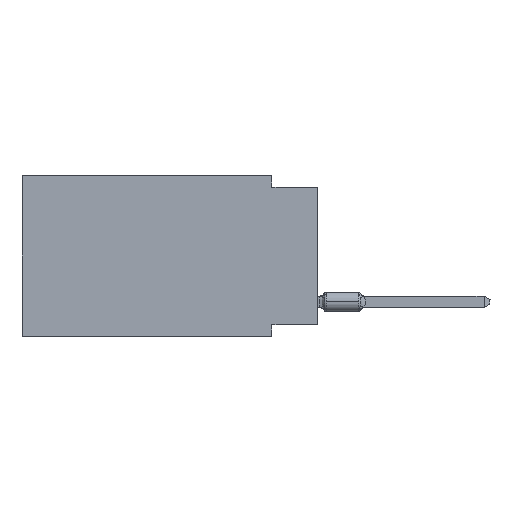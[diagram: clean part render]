
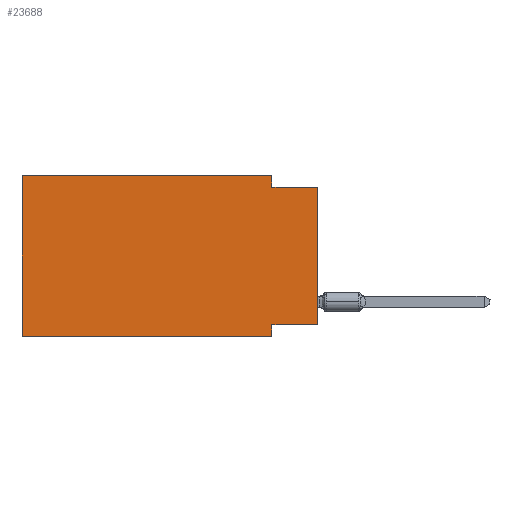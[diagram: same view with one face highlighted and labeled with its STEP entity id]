
A CAD part, left-side view. The second image highlights one B-rep face of the part: STEP entity #23688.
In plain terms, the highlighted planar face has unit normal (-1, 0, 0).
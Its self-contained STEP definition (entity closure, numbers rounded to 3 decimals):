
#523 = LINE ( 'NONE', #6132, #5181 ) ;
#1082 = EDGE_CURVE ( 'NONE', #67866, #2966, #523, .T. ) ;
#2966 = VERTEX_POINT ( 'NONE', #23461 ) ;
#3030 = DIRECTION ( 'NONE',  ( 0., 0., 1. ) ) ;
#3639 = DIRECTION ( 'NONE',  ( 0., 1., 0. ) ) ;
#3882 = VECTOR ( 'NONE', #3030, 1000. ) ;
#4703 = VERTEX_POINT ( 'NONE', #50048 ) ;
#5181 = VECTOR ( 'NONE', #12448, 1000. ) ;
#5575 = EDGE_LOOP ( 'NONE', ( #42075, #51345, #21084, #53376, #48257, #61463, #65077, #19647 ) ) ;
#6132 = CARTESIAN_POINT ( 'NONE',  ( 0., 16.383, 0. ) ) ;
#7193 = AXIS2_PLACEMENT_3D ( 'NONE', #18629, #13002, #58608 ) ;
#8131 = LINE ( 'NONE', #8870, #52992 ) ;
#8870 = CARTESIAN_POINT ( 'NONE',  ( 0., 16.383, 0. ) ) ;
#9353 = CARTESIAN_POINT ( 'NONE',  ( 0., 16.383, 0. ) ) ;
#12448 = DIRECTION ( 'NONE',  ( 0., -1., 0. ) ) ;
#12990 = CARTESIAN_POINT ( 'NONE',  ( 0., 2.54, 0. ) ) ;
#13002 = DIRECTION ( 'NONE',  ( 1., 0., 0. ) ) ;
#13518 = CARTESIAN_POINT ( 'NONE',  ( 0., 2.54, -0.635 ) ) ;
#14638 = EDGE_CURVE ( 'NONE', #60147, #52580, #49582, .T. ) ;
#18629 = CARTESIAN_POINT ( 'NONE',  ( 0., 16.383, 0. ) ) ;
#19647 = ORIENTED_EDGE ( 'NONE', *, *, #14638, .F. ) ;
#21084 = ORIENTED_EDGE ( 'NONE', *, *, #63190, .F. ) ;
#22268 = VECTOR ( 'NONE', #30192, 1000. ) ;
#23461 = CARTESIAN_POINT ( 'NONE',  ( 0., 2.54, 0. ) ) ;
#23688 = ADVANCED_FACE ( 'NONE', ( #30203 ), #41772, .F. ) ;
#24463 = EDGE_CURVE ( 'NONE', #60147, #72265, #46830, .T. ) ;
#25312 = EDGE_CURVE ( 'NONE', #52580, #49282, #31599, .T. ) ;
#26367 = CARTESIAN_POINT ( 'NONE',  ( 0., 2.54, -8.89 ) ) ;
#27574 = CARTESIAN_POINT ( 'NONE',  ( 0., 0., -0.635 ) ) ;
#28910 = VECTOR ( 'NONE', #50147, 1000. ) ;
#30192 = DIRECTION ( 'NONE',  ( 0., 0., -1. ) ) ;
#30203 = FACE_OUTER_BOUND ( 'NONE', #5575, .T. ) ;
#31599 = LINE ( 'NONE', #26367, #43318 ) ;
#32585 = CARTESIAN_POINT ( 'NONE',  ( 0., 16.383, -8.89 ) ) ;
#33531 = DIRECTION ( 'NONE',  ( 0., -1., 0. ) ) ;
#41772 = PLANE ( 'NONE',  #7193 ) ;
#42075 = ORIENTED_EDGE ( 'NONE', *, *, #24463, .T. ) ;
#43318 = VECTOR ( 'NONE', #48796, 1000. ) ;
#46265 = LINE ( 'NONE', #12990, #22268 ) ;
#46830 = LINE ( 'NONE', #58071, #3882 ) ;
#48257 = ORIENTED_EDGE ( 'NONE', *, *, #53502, .F. ) ;
#48796 = DIRECTION ( 'NONE',  ( 0., 0., -1. ) ) ;
#48837 = DIRECTION ( 'NONE',  ( 0., 0., 1. ) ) ;
#49050 = LINE ( 'NONE', #32585, #28910 ) ;
#49282 = VERTEX_POINT ( 'NONE', #66206 ) ;
#49582 = LINE ( 'NONE', #72388, #60807 ) ;
#50048 = CARTESIAN_POINT ( 'NONE',  ( 0., 16.383, -8.89 ) ) ;
#50147 = DIRECTION ( 'NONE',  ( 0., -1., 0. ) ) ;
#51345 = ORIENTED_EDGE ( 'NONE', *, *, #71925, .F. ) ;
#52580 = VERTEX_POINT ( 'NONE', #55951 ) ;
#52992 = VECTOR ( 'NONE', #48837, 1000. ) ;
#53376 = ORIENTED_EDGE ( 'NONE', *, *, #1082, .F. ) ;
#53502 = EDGE_CURVE ( 'NONE', #4703, #67866, #8131, .T. ) ;
#55951 = CARTESIAN_POINT ( 'NONE',  ( 0., 2.54, -8.255 ) ) ;
#56368 = VECTOR ( 'NONE', #33531, 1000. ) ;
#57340 = VERTEX_POINT ( 'NONE', #13518 ) ;
#58071 = CARTESIAN_POINT ( 'NONE',  ( 0., 0., 0. ) ) ;
#58092 = EDGE_CURVE ( 'NONE', #4703, #49282, #49050, .T. ) ;
#58608 = DIRECTION ( 'NONE',  ( 0., 0., -1. ) ) ;
#60147 = VERTEX_POINT ( 'NONE', #66450 ) ;
#60807 = VECTOR ( 'NONE', #3639, 1000. ) ;
#61463 = ORIENTED_EDGE ( 'NONE', *, *, #58092, .T. ) ;
#63190 = EDGE_CURVE ( 'NONE', #2966, #57340, #46265, .T. ) ;
#65077 = ORIENTED_EDGE ( 'NONE', *, *, #25312, .F. ) ;
#65275 = CARTESIAN_POINT ( 'NONE',  ( 0., 0., -0.635 ) ) ;
#66206 = CARTESIAN_POINT ( 'NONE',  ( 0., 2.54, -8.89 ) ) ;
#66450 = CARTESIAN_POINT ( 'NONE',  ( 0., 0., -8.255 ) ) ;
#67866 = VERTEX_POINT ( 'NONE', #9353 ) ;
#67929 = LINE ( 'NONE', #27574, #56368 ) ;
#71925 = EDGE_CURVE ( 'NONE', #57340, #72265, #67929, .T. ) ;
#72265 = VERTEX_POINT ( 'NONE', #65275 ) ;
#72388 = CARTESIAN_POINT ( 'NONE',  ( 0., 0., -8.255 ) ) ;
